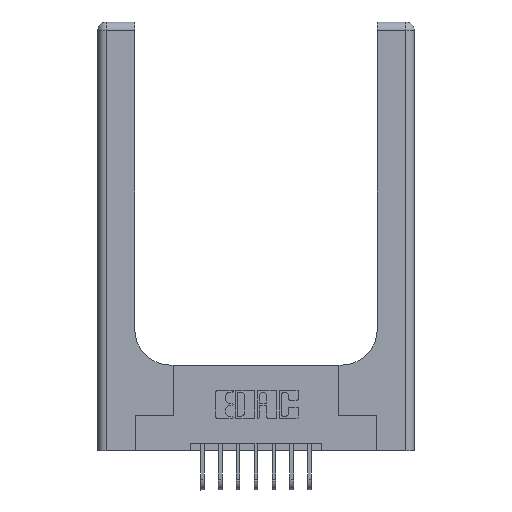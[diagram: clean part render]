
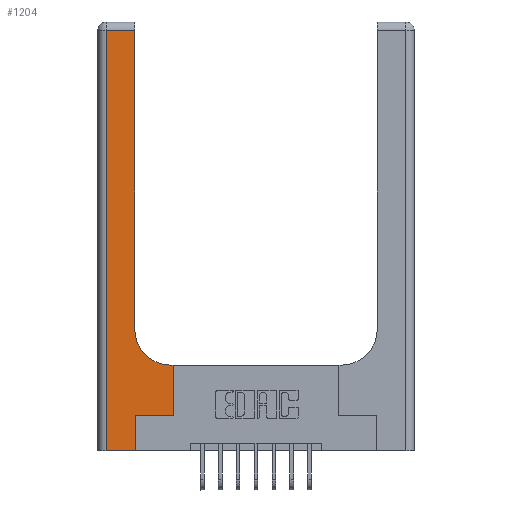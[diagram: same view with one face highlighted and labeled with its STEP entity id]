
A CAD part, top view. The second image highlights one B-rep face of the part: STEP entity #1204.
In plain terms, the highlighted planar face has unit normal (0, 0, 1).
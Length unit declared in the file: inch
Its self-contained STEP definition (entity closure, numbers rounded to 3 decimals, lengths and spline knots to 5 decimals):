
#613 = VECTOR ( 'NONE', #14085, 39.37008 ) ;
#764 = ORIENTED_EDGE ( 'NONE', *, *, #1622, .T. ) ;
#1037 = LINE ( 'NONE', #4746, #15170 ) ;
#1204 = ADVANCED_FACE ( 'NONE', ( #8080 ), #4825, .F. ) ;
#1380 = VERTEX_POINT ( 'NONE', #12719 ) ;
#1396 = CARTESIAN_POINT ( 'NONE',  ( 0.26, 0.85, 0.37 ) ) ;
#1402 = VECTOR ( 'NONE', #12317, 39.37008 ) ;
#1414 = LINE ( 'NONE', #12238, #13829 ) ;
#1470 = VECTOR ( 'NONE', #15699, 39.37008 ) ;
#1499 = EDGE_CURVE ( 'NONE', #2301, #1380, #7656, .T. ) ;
#1544 = CARTESIAN_POINT ( 'NONE',  ( 0., 3., 0.37 ) ) ;
#1622 = EDGE_CURVE ( 'NONE', #12709, #2418, #14980, .T. ) ;
#2200 = AXIS2_PLACEMENT_3D ( 'NONE', #1544, #10333, #11693 ) ;
#2301 = VERTEX_POINT ( 'NONE', #10361 ) ;
#2376 = VECTOR ( 'NONE', #8596, 39.37008 ) ;
#2418 = VERTEX_POINT ( 'NONE', #13195 ) ;
#2657 = CARTESIAN_POINT ( 'NONE',  ( 0.528, 0.6, 0.37 ) ) ;
#2723 = AXIS2_PLACEMENT_3D ( 'NONE', #16261, #3673, #8497 ) ;
#2780 = LINE ( 'NONE', #7995, #2376 ) ;
#2796 = CARTESIAN_POINT ( 'NONE',  ( 0.06, 2.94, 0.37 ) ) ;
#2908 = EDGE_CURVE ( 'NONE', #13015, #13841, #8765, .T. ) ;
#3412 = ORIENTED_EDGE ( 'NONE', *, *, #2908, .T. ) ;
#3656 = CARTESIAN_POINT ( 'NONE',  ( 0.26, 2.94, 0.37 ) ) ;
#3673 = DIRECTION ( 'NONE',  ( 0., 0., -1. ) ) ;
#3887 = CARTESIAN_POINT ( 'NONE',  ( 0.06, 3., 0.37 ) ) ;
#4458 = CARTESIAN_POINT ( 'NONE',  ( 0.51, 0.6, 0.37 ) ) ;
#4691 = DIRECTION ( 'NONE',  ( 1., 0., 0. ) ) ;
#4746 = CARTESIAN_POINT ( 'NONE',  ( 0.26, 0.6, 0.37 ) ) ;
#4825 = PLANE ( 'NONE',  #2200 ) ;
#6135 = EDGE_CURVE ( 'NONE', #1380, #7620, #8136, .T. ) ;
#6872 = LINE ( 'NONE', #7878, #613 ) ;
#7052 = ORIENTED_EDGE ( 'NONE', *, *, #7121, .T. ) ;
#7056 = EDGE_CURVE ( 'NONE', #8255, #13015, #1037, .T. ) ;
#7121 = EDGE_CURVE ( 'NONE', #2418, #2301, #1414, .T. ) ;
#7226 = CARTESIAN_POINT ( 'NONE',  ( 0.265, 0., 0.37 ) ) ;
#7240 = DIRECTION ( 'NONE',  ( -1., 0., 0. ) ) ;
#7620 = VERTEX_POINT ( 'NONE', #9675 ) ;
#7656 = LINE ( 'NONE', #7226, #1402 ) ;
#7878 = CARTESIAN_POINT ( 'NONE',  ( 0., 2.94, 0.37 ) ) ;
#7995 = CARTESIAN_POINT ( 'NONE',  ( 0.528, 0.25, 0.37 ) ) ;
#8080 = FACE_OUTER_BOUND ( 'NONE', #15269, .T. ) ;
#8136 = LINE ( 'NONE', #12014, #1470 ) ;
#8250 = ORIENTED_EDGE ( 'NONE', *, *, #15622, .T. ) ;
#8255 = VERTEX_POINT ( 'NONE', #2657 ) ;
#8497 = DIRECTION ( 'NONE',  ( 1., 0., 0. ) ) ;
#8596 = DIRECTION ( 'NONE',  ( 0., 1., 0. ) ) ;
#8765 = CIRCLE ( 'NONE', #2723, 0.25 ) ;
#9675 = CARTESIAN_POINT ( 'NONE',  ( 0.528, 0.25, 0.37 ) ) ;
#9736 = ORIENTED_EDGE ( 'NONE', *, *, #10318, .T. ) ;
#9794 = ORIENTED_EDGE ( 'NONE', *, *, #9846, .T. ) ;
#9846 = EDGE_CURVE ( 'NONE', #7620, #8255, #2780, .T. ) ;
#10318 = EDGE_CURVE ( 'NONE', #14372, #12709, #6872, .T. ) ;
#10333 = DIRECTION ( 'NONE',  ( 0., 0., -1. ) ) ;
#10361 = CARTESIAN_POINT ( 'NONE',  ( 0.265, 0., 0.37 ) ) ;
#11035 = ORIENTED_EDGE ( 'NONE', *, *, #6135, .T. ) ;
#11207 = VECTOR ( 'NONE', #12690, 39.37008 ) ;
#11693 = DIRECTION ( 'NONE',  ( -1., 0., 0. ) ) ;
#12014 = CARTESIAN_POINT ( 'NONE',  ( 0.265, 0.25, 0.37 ) ) ;
#12238 = CARTESIAN_POINT ( 'NONE',  ( 0., 0., 0.37 ) ) ;
#12317 = DIRECTION ( 'NONE',  ( 0., 1., 0. ) ) ;
#12399 = DIRECTION ( 'NONE',  ( 0., 1., 0. ) ) ;
#12690 = DIRECTION ( 'NONE',  ( 0., -1., 0. ) ) ;
#12709 = VERTEX_POINT ( 'NONE', #2796 ) ;
#12719 = CARTESIAN_POINT ( 'NONE',  ( 0.265, 0.25, 0.37 ) ) ;
#12999 = ORIENTED_EDGE ( 'NONE', *, *, #1499, .T. ) ;
#13015 = VERTEX_POINT ( 'NONE', #4458 ) ;
#13195 = CARTESIAN_POINT ( 'NONE',  ( 0.06, 0., 0.37 ) ) ;
#13471 = VECTOR ( 'NONE', #12399, 39.37008 ) ;
#13636 = ORIENTED_EDGE ( 'NONE', *, *, #7056, .T. ) ;
#13697 = LINE ( 'NONE', #14721, #13471 ) ;
#13829 = VECTOR ( 'NONE', #4691, 39.37008 ) ;
#13841 = VERTEX_POINT ( 'NONE', #1396 ) ;
#14085 = DIRECTION ( 'NONE',  ( -1., 0., 0. ) ) ;
#14372 = VERTEX_POINT ( 'NONE', #3656 ) ;
#14721 = CARTESIAN_POINT ( 'NONE',  ( 0.26, 3., 0.37 ) ) ;
#14980 = LINE ( 'NONE', #3887, #11207 ) ;
#15170 = VECTOR ( 'NONE', #7240, 39.37008 ) ;
#15269 = EDGE_LOOP ( 'NONE', ( #8250, #9736, #764, #7052, #12999, #11035, #9794, #13636, #3412 ) ) ;
#15622 = EDGE_CURVE ( 'NONE', #13841, #14372, #13697, .T. ) ;
#15699 = DIRECTION ( 'NONE',  ( 1., 0., 0. ) ) ;
#16261 = CARTESIAN_POINT ( 'NONE',  ( 0.51, 0.85, 0.37 ) ) ;
